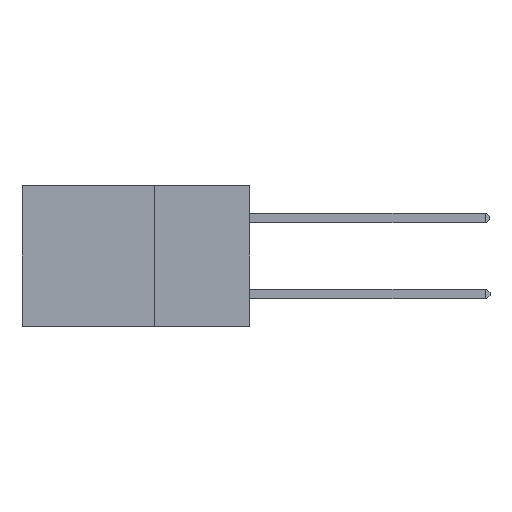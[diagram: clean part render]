
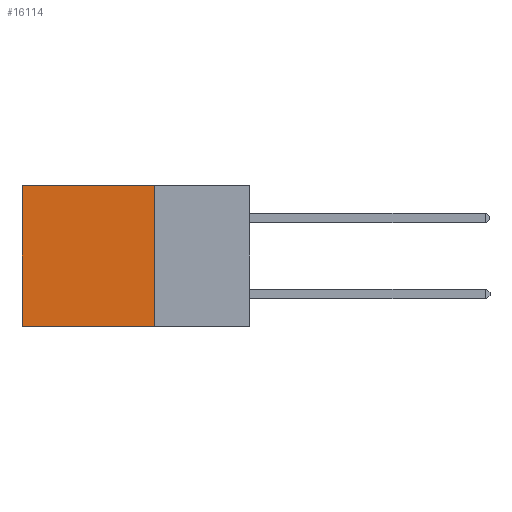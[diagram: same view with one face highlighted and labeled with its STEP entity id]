
A CAD part, left-side view. The second image highlights one B-rep face of the part: STEP entity #16114.
In plain terms, the highlighted planar face has unit normal (-1, 0, 0).
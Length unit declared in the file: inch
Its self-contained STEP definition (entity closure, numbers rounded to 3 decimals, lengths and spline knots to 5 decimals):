
#575 = ORIENTED_EDGE ( 'NONE', *, *, #8497, .F. ) ;
#1503 = LINE ( 'NONE', #3965, #14485 ) ;
#2182 = LINE ( 'NONE', #19866, #6606 ) ;
#2270 = VECTOR ( 'NONE', #13462, 39.37008 ) ;
#3249 = VERTEX_POINT ( 'NONE', #10420 ) ;
#3310 = AXIS2_PLACEMENT_3D ( 'NONE', #16231, #18082, #7215 ) ;
#3740 = EDGE_CURVE ( 'NONE', #4919, #3249, #1503, .T. ) ;
#3965 = CARTESIAN_POINT ( 'NONE',  ( 0.2875, 0.6, 0. ) ) ;
#4919 = VERTEX_POINT ( 'NONE', #18437 ) ;
#5035 = VECTOR ( 'NONE', #5745, 39.37008 ) ;
#5617 = LINE ( 'NONE', #11313, #5035 ) ;
#5745 = DIRECTION ( 'NONE',  ( 0., 1., 0. ) ) ;
#5947 = FACE_OUTER_BOUND ( 'NONE', #14810, .T. ) ;
#6549 = ORIENTED_EDGE ( 'NONE', *, *, #23009, .T. ) ;
#6606 = VECTOR ( 'NONE', #14429, 39.37008 ) ;
#7215 = DIRECTION ( 'NONE',  ( 0., 0., -1. ) ) ;
#8497 = EDGE_CURVE ( 'NONE', #8569, #12194, #2182, .T. ) ;
#8569 = VERTEX_POINT ( 'NONE', #20014 ) ;
#9516 = DIRECTION ( 'NONE',  ( 0., 0., -1. ) ) ;
#9867 = CARTESIAN_POINT ( 'NONE',  ( 0.2875, 0.25, -0.37 ) ) ;
#10420 = CARTESIAN_POINT ( 'NONE',  ( 0.2875, 0.6, -0.37 ) ) ;
#11313 = CARTESIAN_POINT ( 'NONE',  ( 0.2875, 0.25, 0. ) ) ;
#12194 = VERTEX_POINT ( 'NONE', #17457 ) ;
#13462 = DIRECTION ( 'NONE',  ( 0., 1., 0. ) ) ;
#14429 = DIRECTION ( 'NONE',  ( 0., 0., -1. ) ) ;
#14431 = PLANE ( 'NONE',  #3310 ) ;
#14485 = VECTOR ( 'NONE', #9516, 39.37008 ) ;
#14810 = EDGE_LOOP ( 'NONE', ( #18379, #18145, #575, #6549 ) ) ;
#16114 = ADVANCED_FACE ( 'NONE', ( #5947 ), #14431, .F. ) ;
#16231 = CARTESIAN_POINT ( 'NONE',  ( 0.2875, 0.25, 0. ) ) ;
#16895 = LINE ( 'NONE', #9867, #2270 ) ;
#17457 = CARTESIAN_POINT ( 'NONE',  ( 0.2875, 0.25, -0.37 ) ) ;
#18082 = DIRECTION ( 'NONE',  ( 1., 0., 0. ) ) ;
#18145 = ORIENTED_EDGE ( 'NONE', *, *, #19423, .F. ) ;
#18379 = ORIENTED_EDGE ( 'NONE', *, *, #3740, .T. ) ;
#18437 = CARTESIAN_POINT ( 'NONE',  ( 0.2875, 0.6, 0. ) ) ;
#19423 = EDGE_CURVE ( 'NONE', #12194, #3249, #16895, .T. ) ;
#19866 = CARTESIAN_POINT ( 'NONE',  ( 0.2875, 0.25, 0. ) ) ;
#20014 = CARTESIAN_POINT ( 'NONE',  ( 0.2875, 0.25, 0. ) ) ;
#23009 = EDGE_CURVE ( 'NONE', #8569, #4919, #5617, .T. ) ;
